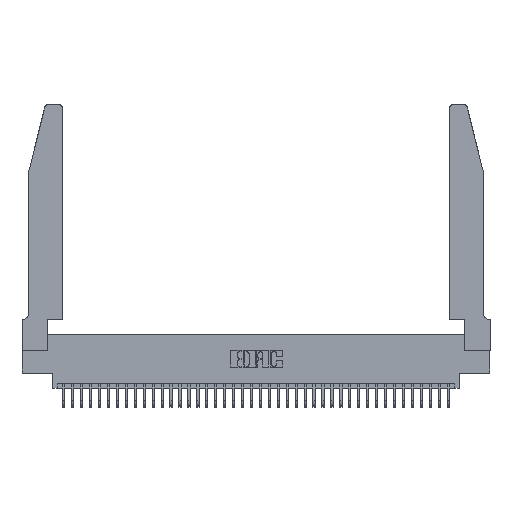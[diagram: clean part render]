
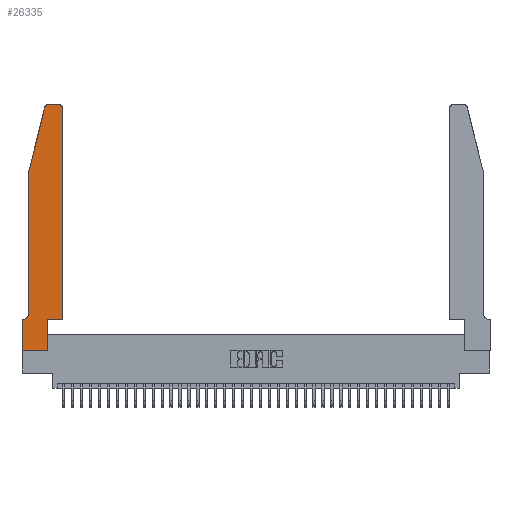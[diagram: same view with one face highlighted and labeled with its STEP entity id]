
A CAD part, top view. The second image highlights one B-rep face of the part: STEP entity #26335.
In plain terms, the highlighted planar face has unit normal (0, 0, 1).
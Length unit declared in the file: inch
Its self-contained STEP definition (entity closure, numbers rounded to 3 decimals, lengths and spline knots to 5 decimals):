
#300 = CARTESIAN_POINT ( 'NONE',  ( 0.0055, 0.42, 0.37 ) ) ;
#311 = ORIENTED_EDGE ( 'NONE', *, *, #15122, .T. ) ;
#593 = VECTOR ( 'NONE', #1223, 39.37008 ) ;
#613 = LINE ( 'NONE', #5174, #6541 ) ;
#671 = CARTESIAN_POINT ( 'NONE',  ( 0.4205, 2.72, 0.37 ) ) ;
#1050 = CARTESIAN_POINT ( 'NONE',  ( 0.0755, 2., 0.37 ) ) ;
#1149 = CARTESIAN_POINT ( 'NONE',  ( 0.4205, 2.75, 0.37 ) ) ;
#1151 = VERTEX_POINT ( 'NONE', #30804 ) ;
#1223 = DIRECTION ( 'NONE',  ( 1., 0., 0. ) ) ;
#1292 = ORIENTED_EDGE ( 'NONE', *, *, #19729, .T. ) ;
#1341 = CARTESIAN_POINT ( 'NONE',  ( 0., 0., 0.37 ) ) ;
#1507 = CARTESIAN_POINT ( 'NONE',  ( 0.25487, 2.72718, 0.37 ) ) ;
#1777 = EDGE_CURVE ( 'NONE', #6792, #1151, #613, .T. ) ;
#3911 = CARTESIAN_POINT ( 'NONE',  ( 0.0755, 0.35, 0.37 ) ) ;
#3929 = CIRCLE ( 'NONE', #27506, 0.03 ) ;
#4310 = CARTESIAN_POINT ( 'NONE',  ( 0., 0.35, 0.37 ) ) ;
#4717 = VERTEX_POINT ( 'NONE', #1149 ) ;
#5174 = CARTESIAN_POINT ( 'NONE',  ( 0.2865, 0.35, 0.37 ) ) ;
#5337 = DIRECTION ( 'NONE',  ( 0., 0., 1. ) ) ;
#5473 = PLANE ( 'NONE',  #24728 ) ;
#5487 = CARTESIAN_POINT ( 'NONE',  ( 0.284, 2.72, 0.37 ) ) ;
#6087 = EDGE_CURVE ( 'NONE', #14379, #15785, #15687, .T. ) ;
#6165 = LINE ( 'NONE', #1050, #38784 ) ;
#6541 = VECTOR ( 'NONE', #27208, 39.37008 ) ;
#6792 = VERTEX_POINT ( 'NONE', #28314 ) ;
#7365 = ORIENTED_EDGE ( 'NONE', *, *, #24813, .T. ) ;
#7678 = VERTEX_POINT ( 'NONE', #23927 ) ;
#8051 = ORIENTED_EDGE ( 'NONE', *, *, #22076, .T. ) ;
#8926 = DIRECTION ( 'NONE',  ( 1., 0., 0. ) ) ;
#9143 = EDGE_CURVE ( 'NONE', #32685, #14379, #32734, .T. ) ;
#9513 = EDGE_LOOP ( 'NONE', ( #36625, #7365, #8051, #21066, #311, #21567, #24360, #27976, #37887, #40044, #9943, #1292 ) ) ;
#9943 = ORIENTED_EDGE ( 'NONE', *, *, #22801, .T. ) ;
#10001 = LINE ( 'NONE', #18215, #36219 ) ;
#10576 = CARTESIAN_POINT ( 'NONE',  ( 0.4505, 0.35, 0.37 ) ) ;
#10631 = DIRECTION ( 'NONE',  ( -0.239, -0.971, 0. ) ) ;
#10938 = CIRCLE ( 'NONE', #34249, 0.03 ) ;
#11268 = CARTESIAN_POINT ( 'NONE',  ( 0., 0., 0.37 ) ) ;
#12925 = DIRECTION ( 'NONE',  ( 0., 0., -1. ) ) ;
#13628 = CARTESIAN_POINT ( 'NONE',  ( 0.0755, 2., 0.37 ) ) ;
#14379 = VERTEX_POINT ( 'NONE', #4310 ) ;
#15122 = EDGE_CURVE ( 'NONE', #30707, #32685, #28295, .T. ) ;
#15167 = VECTOR ( 'NONE', #23332, 39.37008 ) ;
#15687 = LINE ( 'NONE', #1341, #15167 ) ;
#15785 = VERTEX_POINT ( 'NONE', #11268 ) ;
#16100 = EDGE_CURVE ( 'NONE', #15785, #6792, #10001, .T. ) ;
#16658 = CARTESIAN_POINT ( 'NONE',  ( 0.4505, 0.35, 0.37 ) ) ;
#17150 = CARTESIAN_POINT ( 'NONE',  ( 0.0055, 0.35, 0.37 ) ) ;
#17339 = LINE ( 'NONE', #13628, #29743 ) ;
#18215 = CARTESIAN_POINT ( 'NONE',  ( 0., 0., 0.37 ) ) ;
#18554 = VERTEX_POINT ( 'NONE', #1507 ) ;
#18667 = EDGE_CURVE ( 'NONE', #1151, #30103, #36123, .T. ) ;
#18865 = DIRECTION ( 'NONE',  ( -1., 0., 0. ) ) ;
#19729 = EDGE_CURVE ( 'NONE', #19973, #4717, #3929, .T. ) ;
#19973 = VERTEX_POINT ( 'NONE', #20322 ) ;
#20006 = VECTOR ( 'NONE', #18865, 39.37008 ) ;
#20322 = CARTESIAN_POINT ( 'NONE',  ( 0.4505, 2.72, 0.37 ) ) ;
#20793 = DIRECTION ( 'NONE',  ( 0., 1., 0. ) ) ;
#21066 = ORIENTED_EDGE ( 'NONE', *, *, #24480, .T. ) ;
#21292 = AXIS2_PLACEMENT_3D ( 'NONE', #300, #12925, #34902 ) ;
#21567 = ORIENTED_EDGE ( 'NONE', *, *, #9143, .T. ) ;
#21721 = EDGE_CURVE ( 'NONE', #4717, #33441, #28390, .T. ) ;
#22076 = EDGE_CURVE ( 'NONE', #18554, #7678, #6165, .T. ) ;
#22801 = EDGE_CURVE ( 'NONE', #30103, #19973, #32802, .T. ) ;
#22986 = DIRECTION ( 'NONE',  ( 0., -1., 0. ) ) ;
#23332 = DIRECTION ( 'NONE',  ( 0., -1., 0. ) ) ;
#23618 = CARTESIAN_POINT ( 'NONE',  ( 0.4505, 0.35, 0.37 ) ) ;
#23927 = CARTESIAN_POINT ( 'NONE',  ( 0.0755, 2., 0.37 ) ) ;
#24210 = DIRECTION ( 'NONE',  ( 1., 0., 0. ) ) ;
#24360 = ORIENTED_EDGE ( 'NONE', *, *, #6087, .T. ) ;
#24480 = EDGE_CURVE ( 'NONE', #7678, #30707, #17339, .T. ) ;
#24728 = AXIS2_PLACEMENT_3D ( 'NONE', #33895, #5337, #24210 ) ;
#24813 = EDGE_CURVE ( 'NONE', #33441, #18554, #10938, .T. ) ;
#26335 = ADVANCED_FACE ( 'NONE', ( #33336 ), #5473, .T. ) ;
#26833 = CARTESIAN_POINT ( 'NONE',  ( 0.0755, 0.42, 0.37 ) ) ;
#27208 = DIRECTION ( 'NONE',  ( 0., 1., 0. ) ) ;
#27506 = AXIS2_PLACEMENT_3D ( 'NONE', #671, #32084, #35687 ) ;
#27976 = ORIENTED_EDGE ( 'NONE', *, *, #16100, .T. ) ;
#28295 = CIRCLE ( 'NONE', #21292, 0.07 ) ;
#28314 = CARTESIAN_POINT ( 'NONE',  ( 0.2865, 0., 0.37 ) ) ;
#28390 = LINE ( 'NONE', #34658, #20006 ) ;
#29120 = DIRECTION ( 'NONE',  ( -1., 0., 0. ) ) ;
#29244 = VECTOR ( 'NONE', #29120, 39.37008 ) ;
#29743 = VECTOR ( 'NONE', #22986, 39.37008 ) ;
#30103 = VERTEX_POINT ( 'NONE', #16658 ) ;
#30587 = DIRECTION ( 'NONE',  ( 0., 0., 1. ) ) ;
#30707 = VERTEX_POINT ( 'NONE', #26833 ) ;
#30804 = CARTESIAN_POINT ( 'NONE',  ( 0.2865, 0.35, 0.37 ) ) ;
#32084 = DIRECTION ( 'NONE',  ( 0., 0., 1. ) ) ;
#32685 = VERTEX_POINT ( 'NONE', #17150 ) ;
#32734 = LINE ( 'NONE', #3911, #29244 ) ;
#32802 = LINE ( 'NONE', #10576, #34246 ) ;
#33167 = CARTESIAN_POINT ( 'NONE',  ( 0.284, 2.75, 0.37 ) ) ;
#33336 = FACE_OUTER_BOUND ( 'NONE', #9513, .T. ) ;
#33441 = VERTEX_POINT ( 'NONE', #33167 ) ;
#33895 = CARTESIAN_POINT ( 'NONE',  ( 0., 0.35, 0.37 ) ) ;
#34150 = DIRECTION ( 'NONE',  ( 1., 0., 0. ) ) ;
#34246 = VECTOR ( 'NONE', #20793, 39.37008 ) ;
#34249 = AXIS2_PLACEMENT_3D ( 'NONE', #5487, #30587, #8926 ) ;
#34658 = CARTESIAN_POINT ( 'NONE',  ( 0.2605, 2.75, 0.37 ) ) ;
#34902 = DIRECTION ( 'NONE',  ( -1., 0., 0. ) ) ;
#35687 = DIRECTION ( 'NONE',  ( 1., 0., 0. ) ) ;
#36123 = LINE ( 'NONE', #23618, #593 ) ;
#36219 = VECTOR ( 'NONE', #34150, 39.37008 ) ;
#36625 = ORIENTED_EDGE ( 'NONE', *, *, #21721, .T. ) ;
#37887 = ORIENTED_EDGE ( 'NONE', *, *, #1777, .T. ) ;
#38784 = VECTOR ( 'NONE', #10631, 39.37008 ) ;
#40044 = ORIENTED_EDGE ( 'NONE', *, *, #18667, .T. ) ;
